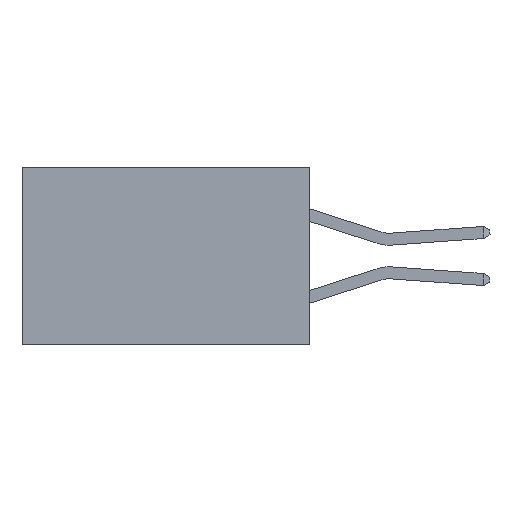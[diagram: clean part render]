
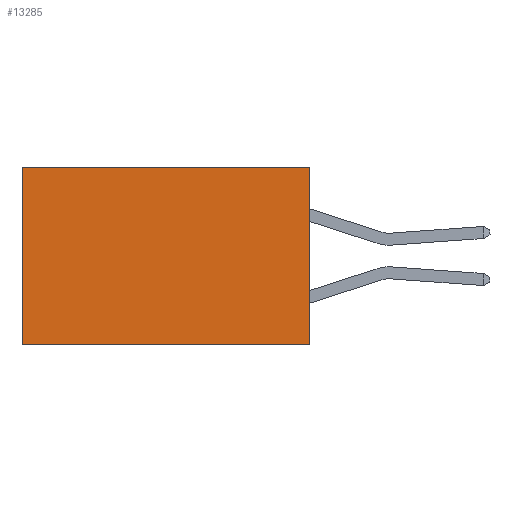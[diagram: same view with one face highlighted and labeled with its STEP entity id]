
A CAD part, left-side view. The second image highlights one B-rep face of the part: STEP entity #13285.
In plain terms, the highlighted planar face has unit normal (-1, 0, 0).
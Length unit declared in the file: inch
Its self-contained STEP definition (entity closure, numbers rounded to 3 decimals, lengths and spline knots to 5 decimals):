
#327 = CARTESIAN_POINT ( 'NONE',  ( 0.298, 0.6, -0.37 ) ) ;
#1801 = CARTESIAN_POINT ( 'NONE',  ( 0.298, 0., -0.37 ) ) ;
#1805 = DIRECTION ( 'NONE',  ( 0., 1., 0. ) ) ;
#3018 = EDGE_CURVE ( 'NONE', #11695, #6422, #9912, .T. ) ;
#3164 = CARTESIAN_POINT ( 'NONE',  ( 0.298, 0., 0. ) ) ;
#4215 = EDGE_CURVE ( 'NONE', #11695, #11407, #15618, .T. ) ;
#5737 = VERTEX_POINT ( 'NONE', #327 ) ;
#6027 = ORIENTED_EDGE ( 'NONE', *, *, #8269, .F. ) ;
#6344 = VECTOR ( 'NONE', #1805, 39.37008 ) ;
#6422 = VERTEX_POINT ( 'NONE', #9141 ) ;
#6958 = ORIENTED_EDGE ( 'NONE', *, *, #3018, .F. ) ;
#7086 = LINE ( 'NONE', #14896, #13306 ) ;
#7381 = EDGE_LOOP ( 'NONE', ( #8659, #6027, #6958, #14193 ) ) ;
#7519 = CARTESIAN_POINT ( 'NONE',  ( 0.298, 0.6, 0. ) ) ;
#7766 = FACE_OUTER_BOUND ( 'NONE', #7381, .T. ) ;
#8269 = EDGE_CURVE ( 'NONE', #6422, #5737, #9928, .T. ) ;
#8659 = ORIENTED_EDGE ( 'NONE', *, *, #14783, .T. ) ;
#8851 = AXIS2_PLACEMENT_3D ( 'NONE', #9619, #9212, #9161 ) ;
#9141 = CARTESIAN_POINT ( 'NONE',  ( 0.298, 0., -0.37 ) ) ;
#9161 = DIRECTION ( 'NONE',  ( 0., 0., -1. ) ) ;
#9212 = DIRECTION ( 'NONE',  ( 1., 0., 0. ) ) ;
#9218 = PLANE ( 'NONE',  #8851 ) ;
#9236 = VECTOR ( 'NONE', #12340, 39.37008 ) ;
#9619 = CARTESIAN_POINT ( 'NONE',  ( 0.298, 0., 0. ) ) ;
#9912 = LINE ( 'NONE', #3164, #16630 ) ;
#9928 = LINE ( 'NONE', #1801, #6344 ) ;
#11407 = VERTEX_POINT ( 'NONE', #7519 ) ;
#11695 = VERTEX_POINT ( 'NONE', #13643 ) ;
#12104 = DIRECTION ( 'NONE',  ( 0., 0., -1. ) ) ;
#12340 = DIRECTION ( 'NONE',  ( 0., 1., 0. ) ) ;
#13285 = ADVANCED_FACE ( 'NONE', ( #7766 ), #9218, .F. ) ;
#13306 = VECTOR ( 'NONE', #16139, 39.37008 ) ;
#13643 = CARTESIAN_POINT ( 'NONE',  ( 0.298, 0., 0. ) ) ;
#14193 = ORIENTED_EDGE ( 'NONE', *, *, #4215, .T. ) ;
#14783 = EDGE_CURVE ( 'NONE', #11407, #5737, #7086, .T. ) ;
#14896 = CARTESIAN_POINT ( 'NONE',  ( 0.298, 0.6, 0. ) ) ;
#14950 = CARTESIAN_POINT ( 'NONE',  ( 0.298, 0., 0. ) ) ;
#15618 = LINE ( 'NONE', #14950, #9236 ) ;
#16139 = DIRECTION ( 'NONE',  ( 0., 0., -1. ) ) ;
#16630 = VECTOR ( 'NONE', #12104, 39.37008 ) ;
